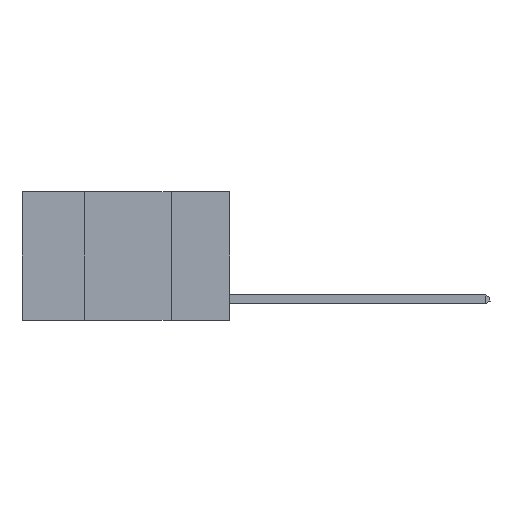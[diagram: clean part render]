
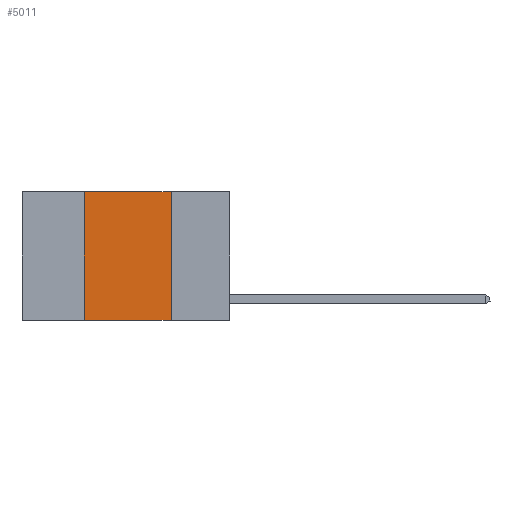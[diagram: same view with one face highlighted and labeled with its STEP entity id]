
A CAD part, left-side view. The second image highlights one B-rep face of the part: STEP entity #5011.
In plain terms, the highlighted planar face has unit normal (-1, 0, 0).
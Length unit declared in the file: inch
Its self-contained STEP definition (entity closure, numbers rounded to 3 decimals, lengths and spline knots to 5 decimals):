
#264 = CARTESIAN_POINT ( 'NONE',  ( 0., 0.17, 0. ) ) ;
#329 = VERTEX_POINT ( 'NONE', #10242 ) ;
#723 = CARTESIAN_POINT ( 'NONE',  ( 0., 0.42, 0. ) ) ;
#1104 = VERTEX_POINT ( 'NONE', #264 ) ;
#1131 = LINE ( 'NONE', #2724, #5663 ) ;
#1716 = ORIENTED_EDGE ( 'NONE', *, *, #3861, .F. ) ;
#2248 = DIRECTION ( 'NONE',  ( 0., -1., 0. ) ) ;
#2724 = CARTESIAN_POINT ( 'NONE',  ( 0., 0.6, -0.37 ) ) ;
#3590 = EDGE_CURVE ( 'NONE', #1104, #4210, #7417, .T. ) ;
#3676 = FACE_OUTER_BOUND ( 'NONE', #6958, .T. ) ;
#3861 = EDGE_CURVE ( 'NONE', #329, #8484, #6876, .T. ) ;
#4210 = VERTEX_POINT ( 'NONE', #9995 ) ;
#5011 = ADVANCED_FACE ( 'NONE', ( #3676 ), #8043, .F. ) ;
#5041 = CARTESIAN_POINT ( 'NONE',  ( 0., 0.17, 0. ) ) ;
#5575 = ORIENTED_EDGE ( 'NONE', *, *, #8035, .F. ) ;
#5663 = VECTOR ( 'NONE', #2248, 39.37008 ) ;
#6161 = DIRECTION ( 'NONE',  ( 0., 0., -1. ) ) ;
#6688 = VECTOR ( 'NONE', #8209, 39.37008 ) ;
#6787 = VECTOR ( 'NONE', #7178, 39.37008 ) ;
#6852 = AXIS2_PLACEMENT_3D ( 'NONE', #8165, #7998, #7952 ) ;
#6876 = LINE ( 'NONE', #723, #6787 ) ;
#6958 = EDGE_LOOP ( 'NONE', ( #8287, #5575, #1716, #8843 ) ) ;
#7178 = DIRECTION ( 'NONE',  ( 0., 0., 1. ) ) ;
#7230 = CARTESIAN_POINT ( 'NONE',  ( 0., 0.42, 0. ) ) ;
#7411 = VECTOR ( 'NONE', #6161, 39.37008 ) ;
#7417 = LINE ( 'NONE', #5041, #7411 ) ;
#7952 = DIRECTION ( 'NONE',  ( 0., 0., -1. ) ) ;
#7998 = DIRECTION ( 'NONE',  ( 1., 0., 0. ) ) ;
#8035 = EDGE_CURVE ( 'NONE', #8484, #1104, #8581, .T. ) ;
#8043 = PLANE ( 'NONE',  #6852 ) ;
#8142 = EDGE_CURVE ( 'NONE', #329, #4210, #1131, .T. ) ;
#8165 = CARTESIAN_POINT ( 'NONE',  ( 0., 0.6, 0. ) ) ;
#8209 = DIRECTION ( 'NONE',  ( 0., -1., 0. ) ) ;
#8287 = ORIENTED_EDGE ( 'NONE', *, *, #3590, .F. ) ;
#8304 = CARTESIAN_POINT ( 'NONE',  ( 0., 0.6, 0. ) ) ;
#8484 = VERTEX_POINT ( 'NONE', #7230 ) ;
#8581 = LINE ( 'NONE', #8304, #6688 ) ;
#8843 = ORIENTED_EDGE ( 'NONE', *, *, #8142, .T. ) ;
#9995 = CARTESIAN_POINT ( 'NONE',  ( 0., 0.17, -0.37 ) ) ;
#10242 = CARTESIAN_POINT ( 'NONE',  ( 0., 0.42, -0.37 ) ) ;
